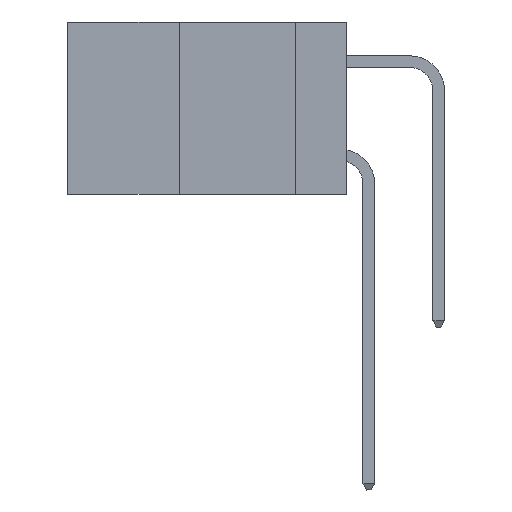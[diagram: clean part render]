
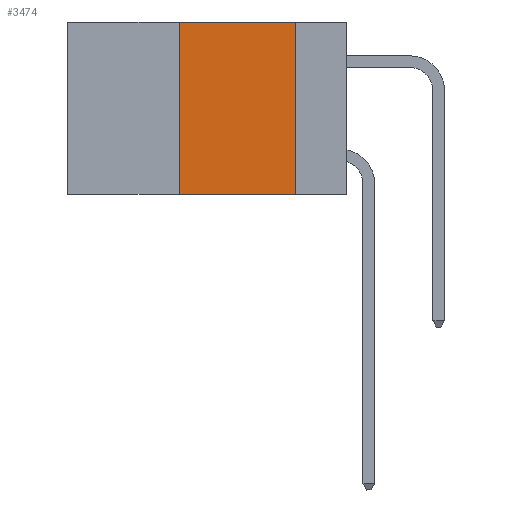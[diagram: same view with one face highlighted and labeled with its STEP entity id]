
A CAD part, left-side view. The second image highlights one B-rep face of the part: STEP entity #3474.
In plain terms, the highlighted planar face has unit normal (-1, 0, 0).
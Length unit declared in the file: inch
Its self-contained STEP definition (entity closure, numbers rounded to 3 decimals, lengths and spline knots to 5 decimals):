
#623 = ORIENTED_EDGE ( 'NONE', *, *, #17661, .F. ) ;
#796 = EDGE_CURVE ( 'NONE', #17795, #13823, #6320, .T. ) ;
#1832 = CARTESIAN_POINT ( 'NONE',  ( 0., 0.6, -0.37 ) ) ;
#3056 = CARTESIAN_POINT ( 'NONE',  ( 0., 0.6, 0. ) ) ;
#3181 = CARTESIAN_POINT ( 'NONE',  ( 0., 0.36, 0. ) ) ;
#3216 = ORIENTED_EDGE ( 'NONE', *, *, #796, .F. ) ;
#3474 = ADVANCED_FACE ( 'NONE', ( #7926 ), #12775, .F. ) ;
#4172 = CARTESIAN_POINT ( 'NONE',  ( 0., 0.11, 0. ) ) ;
#4435 = DIRECTION ( 'NONE',  ( 0., -1., 0. ) ) ;
#4897 = EDGE_LOOP ( 'NONE', ( #17734, #623, #3216, #7329 ) ) ;
#5779 = EDGE_CURVE ( 'NONE', #17795, #11299, #9575, .T. ) ;
#6320 = LINE ( 'NONE', #3181, #7093 ) ;
#7093 = VECTOR ( 'NONE', #8051, 39.37008 ) ;
#7329 = ORIENTED_EDGE ( 'NONE', *, *, #5779, .T. ) ;
#7926 = FACE_OUTER_BOUND ( 'NONE', #4897, .T. ) ;
#8051 = DIRECTION ( 'NONE',  ( 0., 0., 1. ) ) ;
#8055 = CARTESIAN_POINT ( 'NONE',  ( 0., 0.36, -0.37 ) ) ;
#8931 = LINE ( 'NONE', #11639, #18370 ) ;
#9575 = LINE ( 'NONE', #1832, #18789 ) ;
#11299 = VERTEX_POINT ( 'NONE', #19920 ) ;
#11555 = LINE ( 'NONE', #19107, #19507 ) ;
#11639 = CARTESIAN_POINT ( 'NONE',  ( 0., 0.11, 0. ) ) ;
#12215 = DIRECTION ( 'NONE',  ( 0., 0., -1. ) ) ;
#12692 = CARTESIAN_POINT ( 'NONE',  ( 0., 0.36, 0. ) ) ;
#12775 = PLANE ( 'NONE',  #20140 ) ;
#12788 = EDGE_CURVE ( 'NONE', #14278, #11299, #8931, .T. ) ;
#13424 = DIRECTION ( 'NONE',  ( 0., -1., 0. ) ) ;
#13823 = VERTEX_POINT ( 'NONE', #12692 ) ;
#14278 = VERTEX_POINT ( 'NONE', #4172 ) ;
#17661 = EDGE_CURVE ( 'NONE', #13823, #14278, #11555, .T. ) ;
#17734 = ORIENTED_EDGE ( 'NONE', *, *, #12788, .F. ) ;
#17795 = VERTEX_POINT ( 'NONE', #8055 ) ;
#18370 = VECTOR ( 'NONE', #19798, 39.37008 ) ;
#18789 = VECTOR ( 'NONE', #13424, 39.37008 ) ;
#19107 = CARTESIAN_POINT ( 'NONE',  ( 0., 0.6, 0. ) ) ;
#19507 = VECTOR ( 'NONE', #4435, 39.37008 ) ;
#19798 = DIRECTION ( 'NONE',  ( 0., 0., -1. ) ) ;
#19920 = CARTESIAN_POINT ( 'NONE',  ( 0., 0.11, -0.37 ) ) ;
#20140 = AXIS2_PLACEMENT_3D ( 'NONE', #3056, #20518, #12215 ) ;
#20518 = DIRECTION ( 'NONE',  ( 1., 0., 0. ) ) ;
